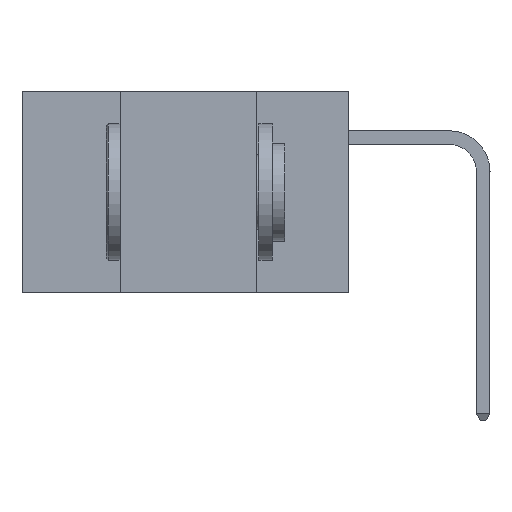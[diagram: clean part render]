
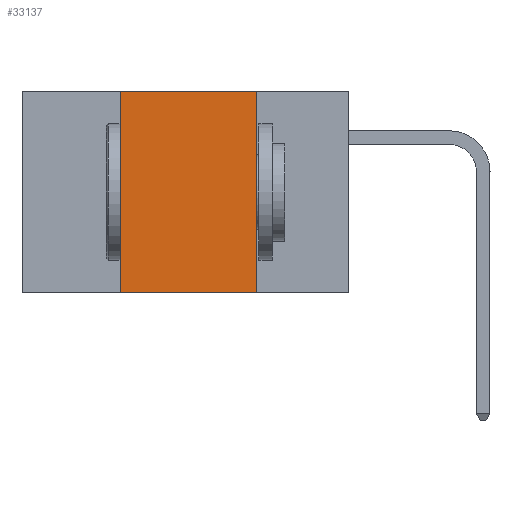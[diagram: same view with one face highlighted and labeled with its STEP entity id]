
A CAD part, left-side view. The second image highlights one B-rep face of the part: STEP entity #33137.
In plain terms, the highlighted planar face has unit normal (-1, 0, 0).
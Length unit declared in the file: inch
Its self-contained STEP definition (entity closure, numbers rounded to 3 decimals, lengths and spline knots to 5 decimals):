
#3484 = CARTESIAN_POINT ( 'NONE',  ( 0., 0.42, -0.37 ) ) ;
#4110 = CARTESIAN_POINT ( 'NONE',  ( 0., 0.6, 0. ) ) ;
#4241 = CARTESIAN_POINT ( 'NONE',  ( 0., 0.17, -0.37 ) ) ;
#4243 = LINE ( 'NONE', #30675, #36816 ) ;
#7398 = DIRECTION ( 'NONE',  ( 0., -1., 0. ) ) ;
#8508 = EDGE_CURVE ( 'NONE', #11437, #10431, #37981, .T. ) ;
#8524 = AXIS2_PLACEMENT_3D ( 'NONE', #18265, #40019, #21424 ) ;
#10308 = ORIENTED_EDGE ( 'NONE', *, *, #19198, .F. ) ;
#10431 = VERTEX_POINT ( 'NONE', #4241 ) ;
#10466 = ORIENTED_EDGE ( 'NONE', *, *, #22660, .F. ) ;
#10541 = ORIENTED_EDGE ( 'NONE', *, *, #10646, .F. ) ;
#10646 = EDGE_CURVE ( 'NONE', #11437, #28582, #4243, .T. ) ;
#10776 = CARTESIAN_POINT ( 'NONE',  ( 0., 0.17, 0. ) ) ;
#10993 = ORIENTED_EDGE ( 'NONE', *, *, #8508, .T. ) ;
#11437 = VERTEX_POINT ( 'NONE', #3484 ) ;
#12208 = LINE ( 'NONE', #4110, #36228 ) ;
#18265 = CARTESIAN_POINT ( 'NONE',  ( 0., 0.6, 0. ) ) ;
#19198 = EDGE_CURVE ( 'NONE', #36010, #10431, #25886, .T. ) ;
#19709 = FACE_OUTER_BOUND ( 'NONE', #37473, .T. ) ;
#21281 = PLANE ( 'NONE',  #8524 ) ;
#21419 = DIRECTION ( 'NONE',  ( 0., 0., 1. ) ) ;
#21424 = DIRECTION ( 'NONE',  ( 0., 0., -1. ) ) ;
#21985 = CARTESIAN_POINT ( 'NONE',  ( 0., 0.6, -0.37 ) ) ;
#22660 = EDGE_CURVE ( 'NONE', #28582, #36010, #12208, .T. ) ;
#24893 = VECTOR ( 'NONE', #27252, 39.37008 ) ;
#25886 = LINE ( 'NONE', #36469, #24893 ) ;
#27252 = DIRECTION ( 'NONE',  ( 0., 0., -1. ) ) ;
#28582 = VERTEX_POINT ( 'NONE', #32812 ) ;
#29751 = VECTOR ( 'NONE', #37606, 39.37008 ) ;
#30675 = CARTESIAN_POINT ( 'NONE',  ( 0., 0.42, 0. ) ) ;
#32812 = CARTESIAN_POINT ( 'NONE',  ( 0., 0.42, 0. ) ) ;
#33137 = ADVANCED_FACE ( 'NONE', ( #19709 ), #21281, .F. ) ;
#36010 = VERTEX_POINT ( 'NONE', #10776 ) ;
#36228 = VECTOR ( 'NONE', #7398, 39.37008 ) ;
#36469 = CARTESIAN_POINT ( 'NONE',  ( 0., 0.17, 0. ) ) ;
#36816 = VECTOR ( 'NONE', #21419, 39.37008 ) ;
#37473 = EDGE_LOOP ( 'NONE', ( #10308, #10466, #10541, #10993 ) ) ;
#37606 = DIRECTION ( 'NONE',  ( 0., -1., 0. ) ) ;
#37981 = LINE ( 'NONE', #21985, #29751 ) ;
#40019 = DIRECTION ( 'NONE',  ( 1., 0., 0. ) ) ;
